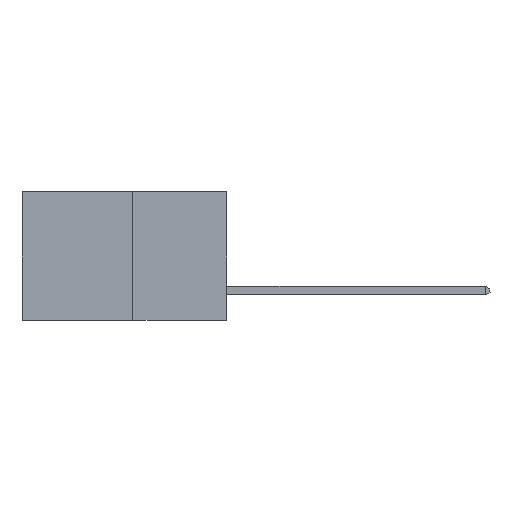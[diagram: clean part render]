
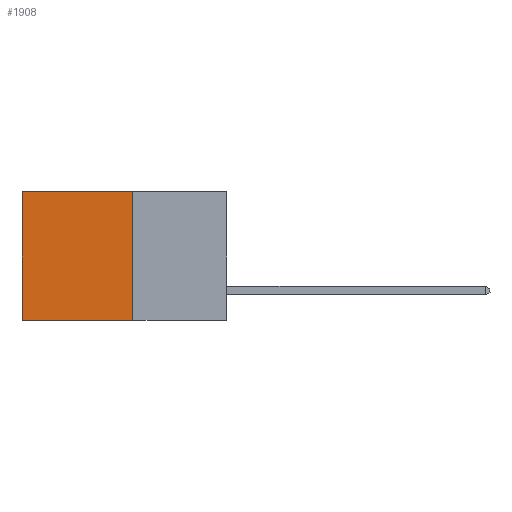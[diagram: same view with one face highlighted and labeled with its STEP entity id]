
A CAD part, left-side view. The second image highlights one B-rep face of the part: STEP entity #1908.
In plain terms, the highlighted planar face has unit normal (-1, 0, 0).
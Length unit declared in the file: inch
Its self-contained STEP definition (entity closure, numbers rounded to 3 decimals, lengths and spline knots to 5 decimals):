
#41 = VERTEX_POINT ( 'NONE', #4763 ) ;
#44 = VECTOR ( 'NONE', #7571, 39.37008 ) ;
#1357 = EDGE_CURVE ( 'NONE', #41, #5143, #6380, .T. ) ;
#1908 = ADVANCED_FACE ( 'NONE', ( #5037 ), #5775, .F. ) ;
#2106 = VECTOR ( 'NONE', #6655, 39.37008 ) ;
#2562 = LINE ( 'NONE', #3454, #8354 ) ;
#3454 = CARTESIAN_POINT ( 'NONE',  ( 0.277, 0.27, 0. ) ) ;
#3605 = DIRECTION ( 'NONE',  ( 0., 1., 0. ) ) ;
#4311 = VERTEX_POINT ( 'NONE', #8988 ) ;
#4373 = AXIS2_PLACEMENT_3D ( 'NONE', #4924, #4498, #6714 ) ;
#4498 = DIRECTION ( 'NONE',  ( 1., 0., 0. ) ) ;
#4595 = LINE ( 'NONE', #5420, #8511 ) ;
#4763 = CARTESIAN_POINT ( 'NONE',  ( 0.277, 0.27, -0.37 ) ) ;
#4924 = CARTESIAN_POINT ( 'NONE',  ( 0.277, 0.27, -0.37 ) ) ;
#5037 = FACE_OUTER_BOUND ( 'NONE', #9498, .T. ) ;
#5143 = VERTEX_POINT ( 'NONE', #8516 ) ;
#5382 = DIRECTION ( 'NONE',  ( 0., 0., -1. ) ) ;
#5420 = CARTESIAN_POINT ( 'NONE',  ( 0.277, 0.27, -0.37 ) ) ;
#5593 = VERTEX_POINT ( 'NONE', #7228 ) ;
#5681 = ORIENTED_EDGE ( 'NONE', *, *, #8045, .T. ) ;
#5775 = PLANE ( 'NONE',  #4373 ) ;
#5816 = ORIENTED_EDGE ( 'NONE', *, *, #1357, .F. ) ;
#5948 = EDGE_CURVE ( 'NONE', #4311, #5593, #2562, .T. ) ;
#6138 = ORIENTED_EDGE ( 'NONE', *, *, #8220, .F. ) ;
#6208 = ORIENTED_EDGE ( 'NONE', *, *, #5948, .T. ) ;
#6380 = LINE ( 'NONE', #8971, #44 ) ;
#6655 = DIRECTION ( 'NONE',  ( 0., 0., -1. ) ) ;
#6714 = DIRECTION ( 'NONE',  ( 0., 0., -1. ) ) ;
#6747 = CARTESIAN_POINT ( 'NONE',  ( 0.277, 0.59, -0.37 ) ) ;
#7228 = CARTESIAN_POINT ( 'NONE',  ( 0.277, 0.59, 0. ) ) ;
#7571 = DIRECTION ( 'NONE',  ( 0., 1., 0. ) ) ;
#7967 = LINE ( 'NONE', #6747, #2106 ) ;
#8045 = EDGE_CURVE ( 'NONE', #5593, #5143, #7967, .T. ) ;
#8220 = EDGE_CURVE ( 'NONE', #4311, #41, #4595, .T. ) ;
#8354 = VECTOR ( 'NONE', #3605, 39.37008 ) ;
#8511 = VECTOR ( 'NONE', #5382, 39.37008 ) ;
#8516 = CARTESIAN_POINT ( 'NONE',  ( 0.277, 0.59, -0.37 ) ) ;
#8971 = CARTESIAN_POINT ( 'NONE',  ( 0.277, 0.27, -0.37 ) ) ;
#8988 = CARTESIAN_POINT ( 'NONE',  ( 0.277, 0.27, 0. ) ) ;
#9498 = EDGE_LOOP ( 'NONE', ( #5681, #5816, #6138, #6208 ) ) ;
